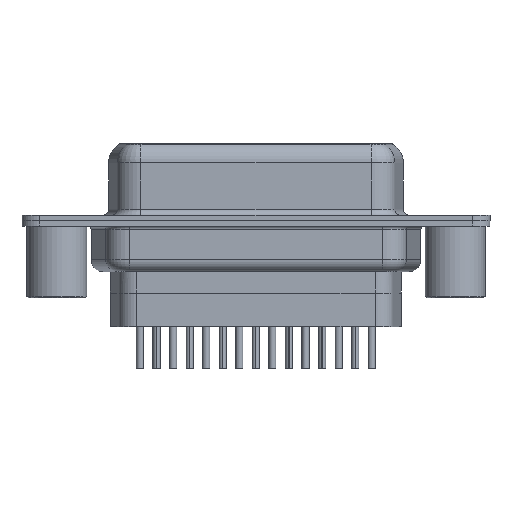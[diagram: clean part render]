
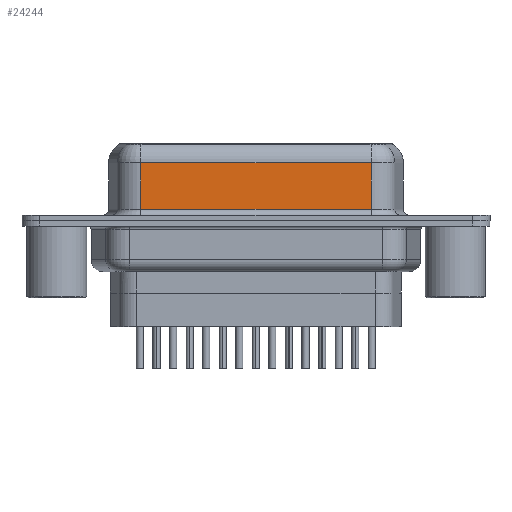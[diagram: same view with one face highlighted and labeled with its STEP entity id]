
A CAD part, front view. The second image highlights one B-rep face of the part: STEP entity #24244.
In plain terms, the highlighted planar face has unit normal (0, -1, 0).
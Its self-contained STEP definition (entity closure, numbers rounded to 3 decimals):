
#1087 = CARTESIAN_POINT ( 'NONE',  ( 7.023, -3.95, 0.95 ) ) ;
#1175 = VERTEX_POINT ( 'NONE', #20016 ) ;
#1443 = FACE_OUTER_BOUND ( 'NONE', #24396, .T. ) ;
#1446 = CARTESIAN_POINT ( 'NONE',  ( 26.297, -3.95, 0.95 ) ) ;
#1470 = CARTESIAN_POINT ( 'NONE',  ( 26.297, -3.95, 4.85 ) ) ;
#2790 = CARTESIAN_POINT ( 'NONE',  ( 26.297, -3.95, 4.85 ) ) ;
#3120 = VECTOR ( 'NONE', #10855, 1000. ) ;
#3323 = EDGE_CURVE ( 'NONE', #14861, #25306, #10617, .T. ) ;
#5016 = VECTOR ( 'NONE', #20820, 1000. ) ;
#6046 = ORIENTED_EDGE ( 'NONE', *, *, #3323, .T. ) ;
#6628 = ORIENTED_EDGE ( 'NONE', *, *, #25568, .T. ) ;
#7520 = DIRECTION ( 'NONE',  ( 0., 0., 1. ) ) ;
#8296 = VECTOR ( 'NONE', #15608, 1000. ) ;
#8906 = DIRECTION ( 'NONE',  ( 0., 0., -1. ) ) ;
#9266 = CARTESIAN_POINT ( 'NONE',  ( 26.297, -3.95, 6.6 ) ) ;
#10469 = CARTESIAN_POINT ( 'NONE',  ( 26.297, -3.95, 0.95 ) ) ;
#10617 = LINE ( 'NONE', #1446, #5016 ) ;
#10855 = DIRECTION ( 'NONE',  ( -1., 0., 0. ) ) ;
#13047 = ORIENTED_EDGE ( 'NONE', *, *, #15284, .T. ) ;
#13617 = CARTESIAN_POINT ( 'NONE',  ( 7.023, -3.95, 6.6 ) ) ;
#14861 = VERTEX_POINT ( 'NONE', #1087 ) ;
#15284 = EDGE_CURVE ( 'NONE', #23840, #1175, #23126, .T. ) ;
#15608 = DIRECTION ( 'NONE',  ( 0., 0., -1. ) ) ;
#16071 = EDGE_CURVE ( 'NONE', #23840, #25306, #18346, .T. ) ;
#17339 = DIRECTION ( 'NONE',  ( 0., 1., 0. ) ) ;
#17959 = AXIS2_PLACEMENT_3D ( 'NONE', #9266, #17339, #7520 ) ;
#18346 = LINE ( 'NONE', #22426, #21235 ) ;
#20016 = CARTESIAN_POINT ( 'NONE',  ( 7.023, -3.95, 4.85 ) ) ;
#20680 = ORIENTED_EDGE ( 'NONE', *, *, #16071, .F. ) ;
#20820 = DIRECTION ( 'NONE',  ( 1., 0., 0. ) ) ;
#21235 = VECTOR ( 'NONE', #8906, 1000. ) ;
#22426 = CARTESIAN_POINT ( 'NONE',  ( 26.297, -3.95, 6.6 ) ) ;
#23126 = LINE ( 'NONE', #2790, #3120 ) ;
#23840 = VERTEX_POINT ( 'NONE', #1470 ) ;
#24244 = ADVANCED_FACE ( 'NONE', ( #1443 ), #25598, .F. ) ;
#24396 = EDGE_LOOP ( 'NONE', ( #20680, #13047, #6628, #6046 ) ) ;
#25306 = VERTEX_POINT ( 'NONE', #10469 ) ;
#25568 = EDGE_CURVE ( 'NONE', #1175, #14861, #25718, .T. ) ;
#25598 = PLANE ( 'NONE',  #17959 ) ;
#25718 = LINE ( 'NONE', #13617, #8296 ) ;
